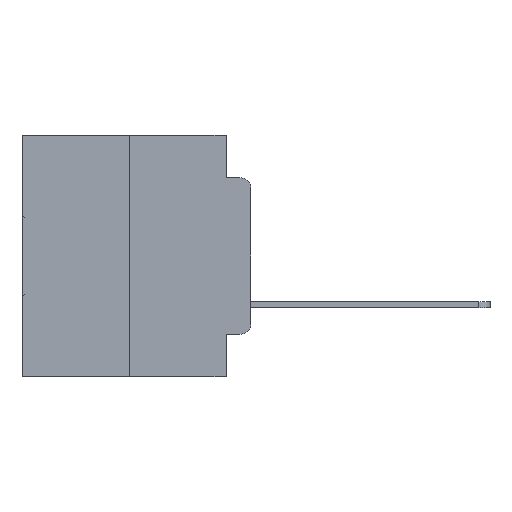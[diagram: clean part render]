
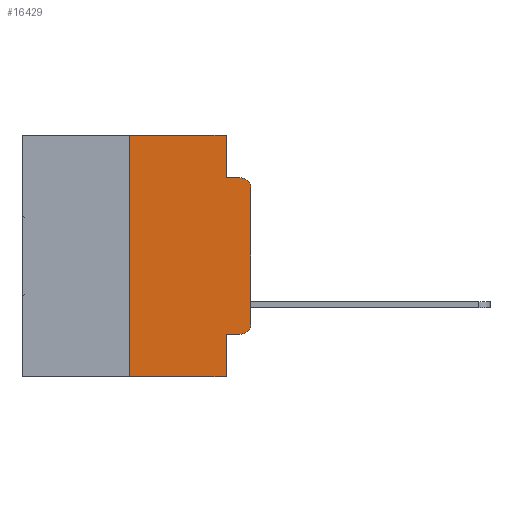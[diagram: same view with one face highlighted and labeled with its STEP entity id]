
A CAD part, left-side view. The second image highlights one B-rep face of the part: STEP entity #16429.
In plain terms, the highlighted planar face has unit normal (-1, 0, 0).
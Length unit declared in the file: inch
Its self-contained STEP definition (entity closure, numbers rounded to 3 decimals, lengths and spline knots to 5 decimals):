
#755 = VERTEX_POINT ( 'NONE', #12722 ) ;
#1116 = CARTESIAN_POINT ( 'NONE',  ( 0., 0.051, -0.0885 ) ) ;
#2532 = VERTEX_POINT ( 'NONE', #7980 ) ;
#5226 = AXIS2_PLACEMENT_3D ( 'NONE', #23531, #8766, #25917 ) ;
#5412 = CARTESIAN_POINT ( 'NONE',  ( 0., 0.25, 0. ) ) ;
#5938 = VERTEX_POINT ( 'NONE', #5412 ) ;
#6104 = VECTOR ( 'NONE', #18438, 39.37008 ) ;
#6160 = PLANE ( 'NONE',  #5226 ) ;
#7112 = EDGE_CURVE ( 'NONE', #5938, #9956, #13596, .T. ) ;
#7458 = DIRECTION ( 'NONE',  ( 0., 0., 1. ) ) ;
#7636 = VECTOR ( 'NONE', #31758, 39.37008 ) ;
#7933 = CARTESIAN_POINT ( 'NONE',  ( 0., 0.02, -0.1085 ) ) ;
#7980 = CARTESIAN_POINT ( 'NONE',  ( 0., 0.02, -0.0885 ) ) ;
#8013 = AXIS2_PLACEMENT_3D ( 'NONE', #7933, #25113, #10378 ) ;
#8517 = VERTEX_POINT ( 'NONE', #1116 ) ;
#8664 = LINE ( 'NONE', #19896, #15322 ) ;
#8766 = DIRECTION ( 'NONE',  ( 1., 0., 0. ) ) ;
#8798 = EDGE_CURVE ( 'NONE', #755, #13485, #20844, .T. ) ;
#9956 = VERTEX_POINT ( 'NONE', #31383 ) ;
#10378 = DIRECTION ( 'NONE',  ( 0., 0., -1. ) ) ;
#11273 = EDGE_CURVE ( 'NONE', #13485, #2532, #27970, .T. ) ;
#11532 = CARTESIAN_POINT ( 'NONE',  ( 0., 0.473, -0.5 ) ) ;
#12441 = DIRECTION ( 'NONE',  ( -1., 0., 0. ) ) ;
#12453 = LINE ( 'NONE', #31189, #24758 ) ;
#12722 = CARTESIAN_POINT ( 'NONE',  ( 0., 0., -0.3915 ) ) ;
#12736 = CARTESIAN_POINT ( 'NONE',  ( 0., 0., 0. ) ) ;
#12924 = VECTOR ( 'NONE', #22526, 39.37008 ) ;
#13465 = DIRECTION ( 'NONE',  ( 0., 0., -1. ) ) ;
#13485 = VERTEX_POINT ( 'NONE', #28386 ) ;
#13565 = CARTESIAN_POINT ( 'NONE',  ( 0., 0.25, -0.5 ) ) ;
#13574 = CARTESIAN_POINT ( 'NONE',  ( 0., 0.051, -0.5 ) ) ;
#13596 = LINE ( 'NONE', #27840, #6104 ) ;
#14080 = DIRECTION ( 'NONE',  ( 0., -1., 0. ) ) ;
#14202 = AXIS2_PLACEMENT_3D ( 'NONE', #26991, #12441, #29286 ) ;
#14375 = CARTESIAN_POINT ( 'NONE',  ( 0., 0.051, -0.0885 ) ) ;
#15177 = CARTESIAN_POINT ( 'NONE',  ( 0., 0.051, 0. ) ) ;
#15322 = VECTOR ( 'NONE', #7458, 39.37008 ) ;
#15843 = VERTEX_POINT ( 'NONE', #13574 ) ;
#16032 = CARTESIAN_POINT ( 'NONE',  ( 0., 0.051, 0. ) ) ;
#16135 = EDGE_CURVE ( 'NONE', #31840, #5938, #8664, .T. ) ;
#16429 = ADVANCED_FACE ( 'NONE', ( #19200 ), #6160, .F. ) ;
#17678 = EDGE_CURVE ( 'NONE', #31840, #15843, #23643, .T. ) ;
#17702 = ORIENTED_EDGE ( 'NONE', *, *, #8798, .T. ) ;
#17734 = ORIENTED_EDGE ( 'NONE', *, *, #11273, .T. ) ;
#17798 = EDGE_CURVE ( 'NONE', #23793, #30250, #12453, .T. ) ;
#18286 = ORIENTED_EDGE ( 'NONE', *, *, #28692, .F. ) ;
#18344 = ORIENTED_EDGE ( 'NONE', *, *, #20273, .F. ) ;
#18438 = DIRECTION ( 'NONE',  ( 0., -1., 0. ) ) ;
#18599 = ORIENTED_EDGE ( 'NONE', *, *, #7112, .F. ) ;
#18658 = ORIENTED_EDGE ( 'NONE', *, *, #16135, .F. ) ;
#18974 = ORIENTED_EDGE ( 'NONE', *, *, #17678, .T. ) ;
#19200 = FACE_OUTER_BOUND ( 'NONE', #27073, .T. ) ;
#19201 = ORIENTED_EDGE ( 'NONE', *, *, #31125, .F. ) ;
#19407 = ORIENTED_EDGE ( 'NONE', *, *, #17798, .T. ) ;
#19446 = EDGE_CURVE ( 'NONE', #30250, #755, #27312, .T. ) ;
#19492 = ORIENTED_EDGE ( 'NONE', *, *, #19446, .T. ) ;
#19581 = LINE ( 'NONE', #15177, #12924 ) ;
#19653 = DIRECTION ( 'NONE',  ( 0., -1., 0. ) ) ;
#19896 = CARTESIAN_POINT ( 'NONE',  ( 0., 0.25, 0. ) ) ;
#20273 = EDGE_CURVE ( 'NONE', #9956, #8517, #19581, .T. ) ;
#20844 = LINE ( 'NONE', #12736, #7636 ) ;
#21880 = LINE ( 'NONE', #14375, #27411 ) ;
#22526 = DIRECTION ( 'NONE',  ( 0., 0., -1. ) ) ;
#23531 = CARTESIAN_POINT ( 'NONE',  ( 0., 0.473, 0. ) ) ;
#23643 = LINE ( 'NONE', #11532, #30446 ) ;
#23793 = VERTEX_POINT ( 'NONE', #30319 ) ;
#24402 = VECTOR ( 'NONE', #13465, 39.37008 ) ;
#24758 = VECTOR ( 'NONE', #19653, 39.37008 ) ;
#24878 = CARTESIAN_POINT ( 'NONE',  ( 0., 0.02, -0.4115 ) ) ;
#25113 = DIRECTION ( 'NONE',  ( -1., 0., 0. ) ) ;
#25917 = DIRECTION ( 'NONE',  ( 0., 0., -1. ) ) ;
#26991 = CARTESIAN_POINT ( 'NONE',  ( 0., 0.02, -0.3915 ) ) ;
#27073 = EDGE_LOOP ( 'NONE', ( #17702, #17734, #18286, #18344, #18599, #18658, #18974, #19201, #19407, #19492 ) ) ;
#27312 = CIRCLE ( 'NONE', #14202, 0.02 ) ;
#27411 = VECTOR ( 'NONE', #30977, 39.37008 ) ;
#27840 = CARTESIAN_POINT ( 'NONE',  ( 0., 0.473, 0. ) ) ;
#27970 = CIRCLE ( 'NONE', #8013, 0.02 ) ;
#28386 = CARTESIAN_POINT ( 'NONE',  ( 0., 0., -0.1085 ) ) ;
#28692 = EDGE_CURVE ( 'NONE', #8517, #2532, #21880, .T. ) ;
#29286 = DIRECTION ( 'NONE',  ( 0., 0., -1. ) ) ;
#30250 = VERTEX_POINT ( 'NONE', #24878 ) ;
#30319 = CARTESIAN_POINT ( 'NONE',  ( 0., 0.051, -0.4115 ) ) ;
#30446 = VECTOR ( 'NONE', #14080, 39.37008 ) ;
#30977 = DIRECTION ( 'NONE',  ( 0., -1., 0. ) ) ;
#31125 = EDGE_CURVE ( 'NONE', #23793, #15843, #31819, .T. ) ;
#31189 = CARTESIAN_POINT ( 'NONE',  ( 0., 0.051, -0.4115 ) ) ;
#31383 = CARTESIAN_POINT ( 'NONE',  ( 0., 0.051, 0. ) ) ;
#31758 = DIRECTION ( 'NONE',  ( 0., 0., 1. ) ) ;
#31819 = LINE ( 'NONE', #16032, #24402 ) ;
#31840 = VERTEX_POINT ( 'NONE', #13565 ) ;
